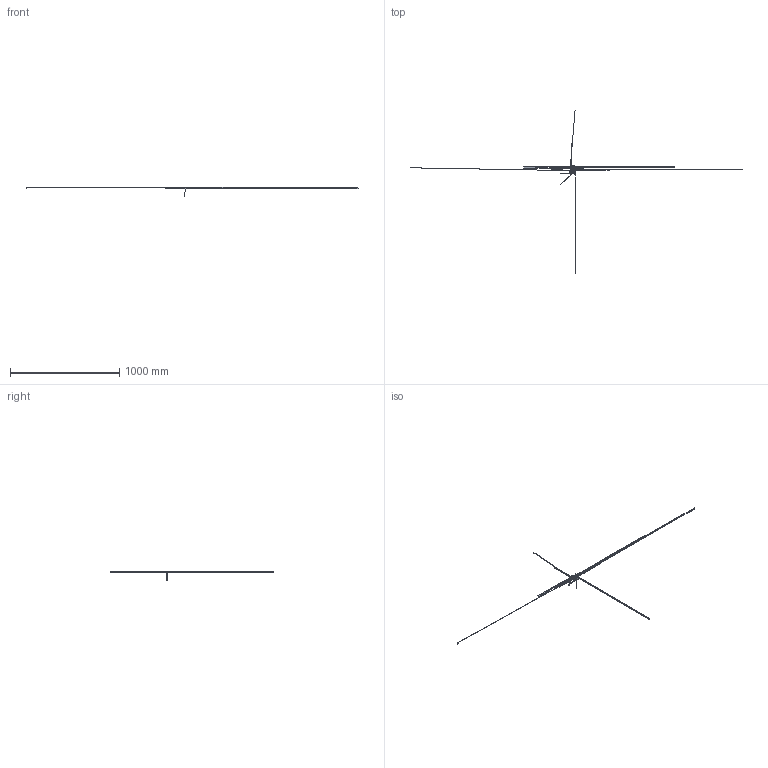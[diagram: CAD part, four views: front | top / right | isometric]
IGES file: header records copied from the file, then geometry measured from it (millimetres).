
Global section: file name: Filename.iges; native system: Open CASCADE 6.5; preprocessor: Open CASCADE IGES processor 6.5; author: ohammer; date: 20130223.112835; units: millimetre
Bounding box: 3033.69 x 1492.97 x 89.82 mm (x, y, z)
Surface area: 54427.4 mm2 (no closed solid volume)
Topology: 0 solids, 0 shells, 141 faces, 774 edges, 772 vertices
Faces by surface type: extrusion 100, bspline 37, revolution 4
